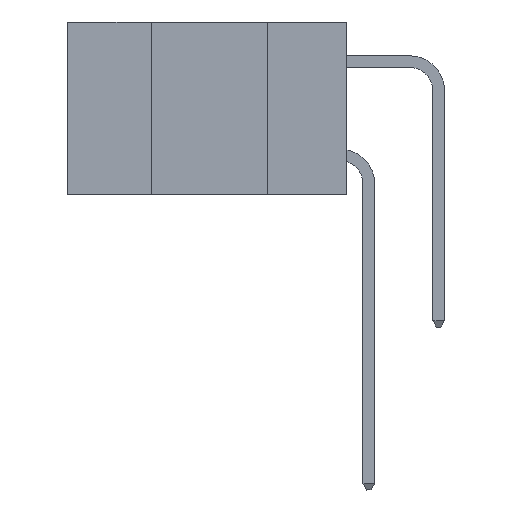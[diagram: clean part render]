
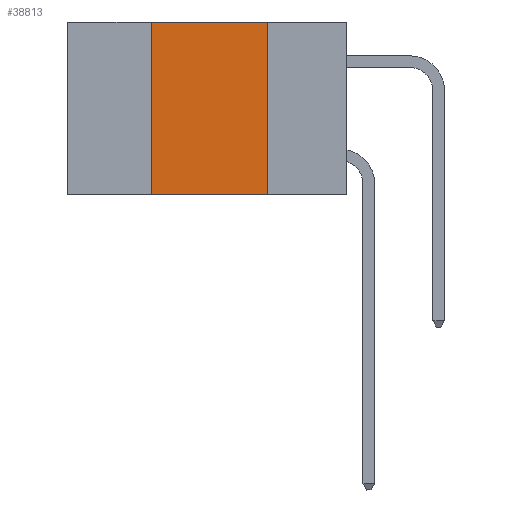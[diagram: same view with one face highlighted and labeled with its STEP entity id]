
A CAD part, left-side view. The second image highlights one B-rep face of the part: STEP entity #38813.
In plain terms, the highlighted planar face has unit normal (-1, 0, 0).
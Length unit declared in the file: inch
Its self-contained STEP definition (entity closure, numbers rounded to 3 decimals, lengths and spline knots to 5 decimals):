
#1181 = VERTEX_POINT ( 'NONE', #34372 ) ;
#1808 = CARTESIAN_POINT ( 'NONE',  ( 0., 0.6, -0.37 ) ) ;
#2600 = CARTESIAN_POINT ( 'NONE',  ( 0., 0.17, -0.37 ) ) ;
#3335 = VERTEX_POINT ( 'NONE', #29186 ) ;
#5706 = ORIENTED_EDGE ( 'NONE', *, *, #24965, .F. ) ;
#6429 = VERTEX_POINT ( 'NONE', #2600 ) ;
#6620 = VECTOR ( 'NONE', #24140, 39.37008 ) ;
#6984 = EDGE_LOOP ( 'NONE', ( #5706, #23982, #10781, #13219 ) ) ;
#9368 = VECTOR ( 'NONE', #17978, 39.37008 ) ;
#9418 = CARTESIAN_POINT ( 'NONE',  ( 0., 0.6, 0. ) ) ;
#9566 = LINE ( 'NONE', #39487, #6620 ) ;
#10781 = ORIENTED_EDGE ( 'NONE', *, *, #21038, .F. ) ;
#13219 = ORIENTED_EDGE ( 'NONE', *, *, #21421, .T. ) ;
#13688 = CARTESIAN_POINT ( 'NONE',  ( 0., 0.17, 0. ) ) ;
#14275 = VECTOR ( 'NONE', #36771, 39.37008 ) ;
#15256 = DIRECTION ( 'NONE',  ( 0., 0., -1. ) ) ;
#15532 = PLANE ( 'NONE',  #22403 ) ;
#16792 = VECTOR ( 'NONE', #23430, 39.37008 ) ;
#17978 = DIRECTION ( 'NONE',  ( 0., 0., -1. ) ) ;
#18284 = EDGE_CURVE ( 'NONE', #3335, #34713, #30707, .T. ) ;
#19690 = LINE ( 'NONE', #1808, #16792 ) ;
#21038 = EDGE_CURVE ( 'NONE', #1181, #3335, #9566, .T. ) ;
#21421 = EDGE_CURVE ( 'NONE', #1181, #6429, #19690, .T. ) ;
#22403 = AXIS2_PLACEMENT_3D ( 'NONE', #30641, #33724, #15256 ) ;
#23430 = DIRECTION ( 'NONE',  ( 0., -1., 0. ) ) ;
#23982 = ORIENTED_EDGE ( 'NONE', *, *, #18284, .F. ) ;
#24140 = DIRECTION ( 'NONE',  ( 0., 0., 1. ) ) ;
#24965 = EDGE_CURVE ( 'NONE', #34713, #6429, #38823, .T. ) ;
#29186 = CARTESIAN_POINT ( 'NONE',  ( 0., 0.42, 0. ) ) ;
#30641 = CARTESIAN_POINT ( 'NONE',  ( 0., 0.6, 0. ) ) ;
#30707 = LINE ( 'NONE', #9418, #14275 ) ;
#33724 = DIRECTION ( 'NONE',  ( 1., 0., 0. ) ) ;
#34372 = CARTESIAN_POINT ( 'NONE',  ( 0., 0.42, -0.37 ) ) ;
#34713 = VERTEX_POINT ( 'NONE', #13688 ) ;
#36225 = FACE_OUTER_BOUND ( 'NONE', #6984, .T. ) ;
#36771 = DIRECTION ( 'NONE',  ( 0., -1., 0. ) ) ;
#38813 = ADVANCED_FACE ( 'NONE', ( #36225 ), #15532, .F. ) ;
#38823 = LINE ( 'NONE', #39398, #9368 ) ;
#39398 = CARTESIAN_POINT ( 'NONE',  ( 0., 0.17, 0. ) ) ;
#39487 = CARTESIAN_POINT ( 'NONE',  ( 0., 0.42, 0. ) ) ;
